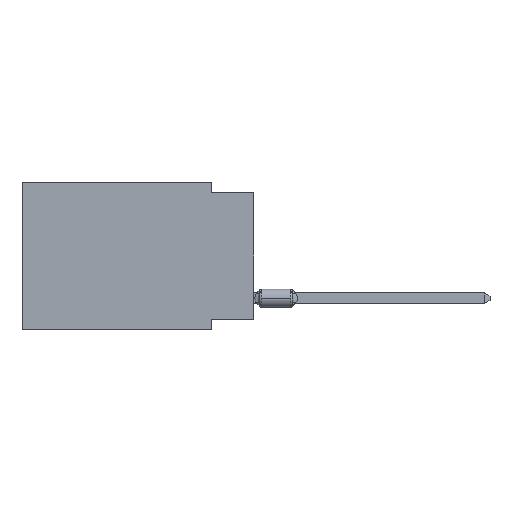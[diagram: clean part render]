
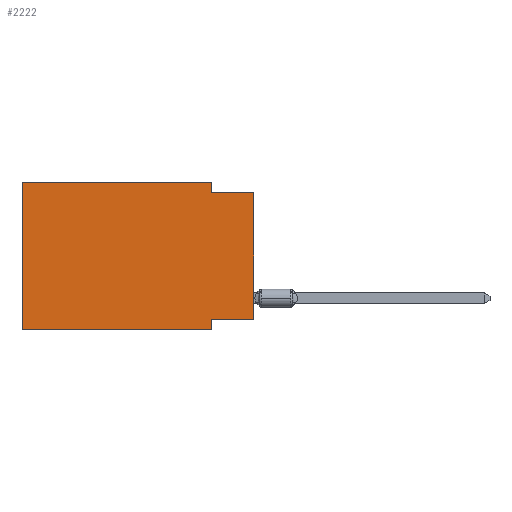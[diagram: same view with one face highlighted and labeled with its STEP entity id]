
A CAD part, left-side view. The second image highlights one B-rep face of the part: STEP entity #2222.
In plain terms, the highlighted planar face has unit normal (-1, 0, 0).
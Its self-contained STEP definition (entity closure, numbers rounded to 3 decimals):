
#170 = AXIS2_PLACEMENT_3D ( 'NONE', #9501, #3060, #2981 ) ;
#1135 = CARTESIAN_POINT ( 'NONE',  ( 0., 0., -0.635 ) ) ;
#1559 = FACE_OUTER_BOUND ( 'NONE', #8492, .T. ) ;
#1586 = ORIENTED_EDGE ( 'NONE', *, *, #13838, .F. ) ;
#1711 = DIRECTION ( 'NONE',  ( 0., 0., 1. ) ) ;
#1897 = ORIENTED_EDGE ( 'NONE', *, *, #15576, .F. ) ;
#2222 = ADVANCED_FACE ( 'NONE', ( #1559 ), #9245, .F. ) ;
#2275 = LINE ( 'NONE', #6120, #16225 ) ;
#2981 = DIRECTION ( 'NONE',  ( 0., 0., -1. ) ) ;
#3060 = DIRECTION ( 'NONE',  ( 1., 0., 0. ) ) ;
#3451 = VERTEX_POINT ( 'NONE', #7368 ) ;
#3480 = EDGE_CURVE ( 'NONE', #12684, #11850, #7213, .T. ) ;
#3500 = EDGE_CURVE ( 'NONE', #13879, #11850, #2275, .T. ) ;
#4066 = ORIENTED_EDGE ( 'NONE', *, *, #11963, .F. ) ;
#4333 = EDGE_CURVE ( 'NONE', #11377, #3451, #8659, .T. ) ;
#4572 = LINE ( 'NONE', #12275, #12461 ) ;
#4692 = CARTESIAN_POINT ( 'NONE',  ( 0., 0., -0.635 ) ) ;
#4767 = VECTOR ( 'NONE', #14814, 1000. ) ;
#5128 = LINE ( 'NONE', #15676, #10864 ) ;
#5223 = VECTOR ( 'NONE', #10120, 1000. ) ;
#5733 = DIRECTION ( 'NONE',  ( 0., 0., 1. ) ) ;
#5755 = VECTOR ( 'NONE', #16325, 1000. ) ;
#5834 = DIRECTION ( 'NONE',  ( 0., 0., -1. ) ) ;
#5914 = DIRECTION ( 'NONE',  ( 0., -1., 0. ) ) ;
#6120 = CARTESIAN_POINT ( 'NONE',  ( 0., 13.97, -8.89 ) ) ;
#6615 = CARTESIAN_POINT ( 'NONE',  ( 0., 2.54, -8.255 ) ) ;
#6687 = ORIENTED_EDGE ( 'NONE', *, *, #3480, .F. ) ;
#6864 = CARTESIAN_POINT ( 'NONE',  ( 0., 0., -8.255 ) ) ;
#7163 = VERTEX_POINT ( 'NONE', #1135 ) ;
#7189 = EDGE_CURVE ( 'NONE', #9017, #7163, #9509, .T. ) ;
#7213 = LINE ( 'NONE', #13644, #5755 ) ;
#7368 = CARTESIAN_POINT ( 'NONE',  ( 0., 2.54, 0. ) ) ;
#7437 = LINE ( 'NONE', #12535, #5223 ) ;
#7734 = CARTESIAN_POINT ( 'NONE',  ( 0., 13.97, -8.89 ) ) ;
#8492 = EDGE_LOOP ( 'NONE', ( #10236, #1897, #4066, #13147, #1586, #15946, #6687, #10179 ) ) ;
#8659 = LINE ( 'NONE', #13681, #14858 ) ;
#9017 = VERTEX_POINT ( 'NONE', #6864 ) ;
#9245 = PLANE ( 'NONE',  #170 ) ;
#9501 = CARTESIAN_POINT ( 'NONE',  ( 0., 13.97, 0. ) ) ;
#9509 = LINE ( 'NONE', #14615, #13628 ) ;
#10120 = DIRECTION ( 'NONE',  ( 0., 1., 0. ) ) ;
#10142 = CARTESIAN_POINT ( 'NONE',  ( 0., 13.97, 0. ) ) ;
#10179 = ORIENTED_EDGE ( 'NONE', *, *, #11804, .F. ) ;
#10236 = ORIENTED_EDGE ( 'NONE', *, *, #7189, .T. ) ;
#10864 = VECTOR ( 'NONE', #1711, 1000. ) ;
#11054 = DIRECTION ( 'NONE',  ( 0., -1., 0. ) ) ;
#11377 = VERTEX_POINT ( 'NONE', #10142 ) ;
#11804 = EDGE_CURVE ( 'NONE', #9017, #12684, #7437, .T. ) ;
#11850 = VERTEX_POINT ( 'NONE', #12777 ) ;
#11963 = EDGE_CURVE ( 'NONE', #3451, #12426, #4572, .T. ) ;
#12275 = CARTESIAN_POINT ( 'NONE',  ( 0., 2.54, 0. ) ) ;
#12318 = CARTESIAN_POINT ( 'NONE',  ( 0., 2.54, -0.635 ) ) ;
#12426 = VERTEX_POINT ( 'NONE', #12318 ) ;
#12461 = VECTOR ( 'NONE', #5834, 1000. ) ;
#12535 = CARTESIAN_POINT ( 'NONE',  ( 0., 0., -8.255 ) ) ;
#12684 = VERTEX_POINT ( 'NONE', #6615 ) ;
#12777 = CARTESIAN_POINT ( 'NONE',  ( 0., 2.54, -8.89 ) ) ;
#13147 = ORIENTED_EDGE ( 'NONE', *, *, #4333, .F. ) ;
#13628 = VECTOR ( 'NONE', #5733, 1000. ) ;
#13644 = CARTESIAN_POINT ( 'NONE',  ( 0., 2.54, -8.89 ) ) ;
#13646 = LINE ( 'NONE', #4692, #4767 ) ;
#13681 = CARTESIAN_POINT ( 'NONE',  ( 0., 13.97, 0. ) ) ;
#13838 = EDGE_CURVE ( 'NONE', #13879, #11377, #5128, .T. ) ;
#13879 = VERTEX_POINT ( 'NONE', #7734 ) ;
#14615 = CARTESIAN_POINT ( 'NONE',  ( 0., 0., 0. ) ) ;
#14814 = DIRECTION ( 'NONE',  ( 0., -1., 0. ) ) ;
#14858 = VECTOR ( 'NONE', #5914, 1000. ) ;
#15576 = EDGE_CURVE ( 'NONE', #12426, #7163, #13646, .T. ) ;
#15676 = CARTESIAN_POINT ( 'NONE',  ( 0., 13.97, 0. ) ) ;
#15946 = ORIENTED_EDGE ( 'NONE', *, *, #3500, .T. ) ;
#16225 = VECTOR ( 'NONE', #11054, 1000. ) ;
#16325 = DIRECTION ( 'NONE',  ( 0., 0., -1. ) ) ;
